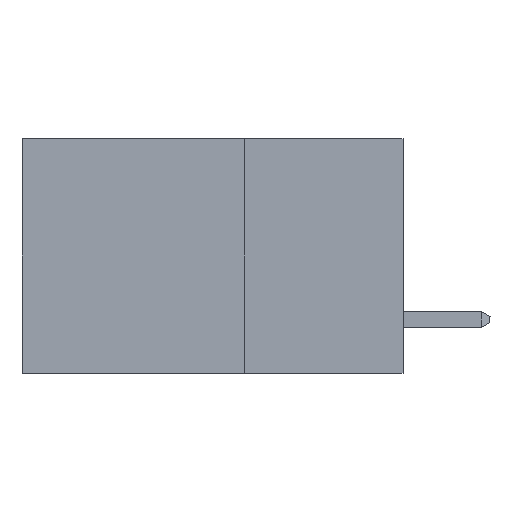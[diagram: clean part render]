
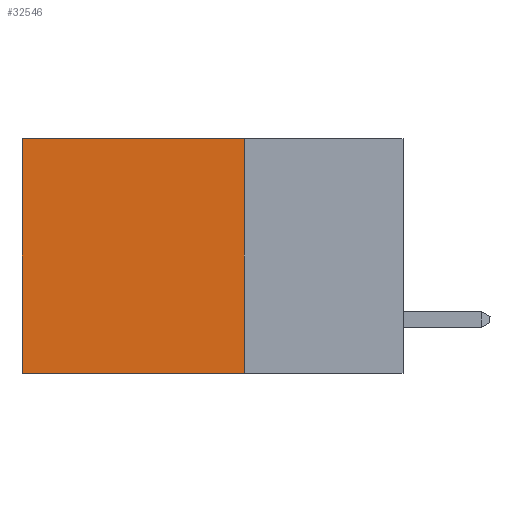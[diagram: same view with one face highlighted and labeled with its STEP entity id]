
A CAD part, left-side view. The second image highlights one B-rep face of the part: STEP entity #32546.
In plain terms, the highlighted planar face has unit normal (-1, 0, 0).
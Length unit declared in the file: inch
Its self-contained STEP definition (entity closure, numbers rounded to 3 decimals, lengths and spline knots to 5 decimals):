
#1156 = EDGE_CURVE ( 'NONE', #45635, #40464, #13676, .T. ) ;
#1966 = CARTESIAN_POINT ( 'NONE',  ( 0.2875, 0.25, 0. ) ) ;
#2578 = LINE ( 'NONE', #1966, #28659 ) ;
#4014 = PLANE ( 'NONE',  #39158 ) ;
#5540 = EDGE_LOOP ( 'NONE', ( #29109, #6817, #42218, #22785 ) ) ;
#6101 = DIRECTION ( 'NONE',  ( 0., 1., 0. ) ) ;
#6654 = DIRECTION ( 'NONE',  ( 0., 0., -1. ) ) ;
#6671 = DIRECTION ( 'NONE',  ( 0., 0., -1. ) ) ;
#6719 = EDGE_CURVE ( 'NONE', #21356, #40464, #7399, .T. ) ;
#6817 = ORIENTED_EDGE ( 'NONE', *, *, #6719, .F. ) ;
#7310 = VECTOR ( 'NONE', #6671, 39.37008 ) ;
#7399 = LINE ( 'NONE', #46913, #11936 ) ;
#8276 = EDGE_CURVE ( 'NONE', #40118, #21356, #42491, .T. ) ;
#11936 = VECTOR ( 'NONE', #43850, 39.37008 ) ;
#13676 = LINE ( 'NONE', #21083, #30732 ) ;
#15386 = DIRECTION ( 'NONE',  ( 0., 0., -1. ) ) ;
#18794 = CARTESIAN_POINT ( 'NONE',  ( 0.2875, 0.6, 0. ) ) ;
#21083 = CARTESIAN_POINT ( 'NONE',  ( 0.2875, 0.6, 0. ) ) ;
#21356 = VERTEX_POINT ( 'NONE', #28380 ) ;
#22785 = ORIENTED_EDGE ( 'NONE', *, *, #33406, .T. ) ;
#23126 = FACE_OUTER_BOUND ( 'NONE', #5540, .T. ) ;
#26213 = DIRECTION ( 'NONE',  ( 1., 0., 0. ) ) ;
#26408 = CARTESIAN_POINT ( 'NONE',  ( 0.2875, 0.25, 0. ) ) ;
#28380 = CARTESIAN_POINT ( 'NONE',  ( 0.2875, 0.25, -0.37 ) ) ;
#28659 = VECTOR ( 'NONE', #6101, 39.37008 ) ;
#29109 = ORIENTED_EDGE ( 'NONE', *, *, #1156, .T. ) ;
#30732 = VECTOR ( 'NONE', #6654, 39.37008 ) ;
#30913 = CARTESIAN_POINT ( 'NONE',  ( 0.2875, 0.6, -0.37 ) ) ;
#32546 = ADVANCED_FACE ( 'NONE', ( #23126 ), #4014, .F. ) ;
#33406 = EDGE_CURVE ( 'NONE', #40118, #45635, #2578, .T. ) ;
#38624 = CARTESIAN_POINT ( 'NONE',  ( 0.2875, 0.25, 0. ) ) ;
#39158 = AXIS2_PLACEMENT_3D ( 'NONE', #44301, #26213, #15386 ) ;
#40118 = VERTEX_POINT ( 'NONE', #38624 ) ;
#40464 = VERTEX_POINT ( 'NONE', #30913 ) ;
#42218 = ORIENTED_EDGE ( 'NONE', *, *, #8276, .F. ) ;
#42491 = LINE ( 'NONE', #26408, #7310 ) ;
#43850 = DIRECTION ( 'NONE',  ( 0., 1., 0. ) ) ;
#44301 = CARTESIAN_POINT ( 'NONE',  ( 0.2875, 0.25, 0. ) ) ;
#45635 = VERTEX_POINT ( 'NONE', #18794 ) ;
#46913 = CARTESIAN_POINT ( 'NONE',  ( 0.2875, 0.25, -0.37 ) ) ;
